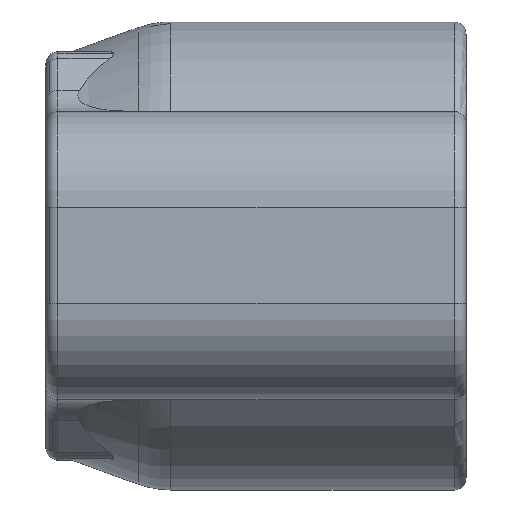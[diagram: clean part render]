
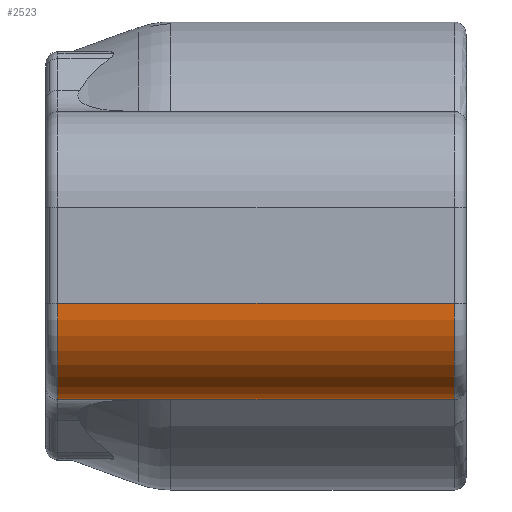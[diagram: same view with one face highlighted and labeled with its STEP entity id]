
A CAD part, top view. The second image highlights one B-rep face of the part: STEP entity #2523.
In plain terms, the highlighted cylindrical face has radius 8 mm (diameter 16 mm), a partial arc.
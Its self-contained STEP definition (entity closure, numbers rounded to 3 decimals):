
#264 = DIRECTION ( 'NONE',  ( 0., 0., 1. ) ) ;
#381 = VERTEX_POINT ( 'NONE', #6163 ) ;
#621 = EDGE_CURVE ( 'NONE', #2818, #786, #5773, .T. ) ;
#786 = VERTEX_POINT ( 'NONE', #4463 ) ;
#959 = FACE_OUTER_BOUND ( 'NONE', #5368, .T. ) ;
#1476 = AXIS2_PLACEMENT_3D ( 'NONE', #1784, #1839, #2491 ) ;
#1775 = AXIS2_PLACEMENT_3D ( 'NONE', #8683, #5584, #264 ) ;
#1784 = CARTESIAN_POINT ( 'NONE',  ( 164.981, -4., -79. ) ) ;
#1839 = DIRECTION ( 'NONE',  ( -1., 0., 0. ) ) ;
#2408 = DIRECTION ( 'NONE',  ( 1., 0., 0. ) ) ;
#2491 = DIRECTION ( 'NONE',  ( 0., 0., -1. ) ) ;
#2497 = VERTEX_POINT ( 'NONE', #4099 ) ;
#2523 = ADVANCED_FACE ( 'NONE', ( #959 ), #3412, .T. ) ;
#2673 = EDGE_CURVE ( 'NONE', #381, #2497, #6860, .T. ) ;
#2765 = CARTESIAN_POINT ( 'NONE',  ( 131.981, -4., -79. ) ) ;
#2818 = VERTEX_POINT ( 'NONE', #5273 ) ;
#2853 = VECTOR ( 'NONE', #9043, 1000. ) ;
#3150 = EDGE_CURVE ( 'NONE', #381, #2818, #9167, .T. ) ;
#3412 = CYLINDRICAL_SURFACE ( 'NONE', #1775, 8. ) ;
#4099 = CARTESIAN_POINT ( 'NONE',  ( 131.981, -4., -71. ) ) ;
#4325 = AXIS2_PLACEMENT_3D ( 'NONE', #2765, #8084, #9570 ) ;
#4463 = CARTESIAN_POINT ( 'NONE',  ( 164.981, -4., -71. ) ) ;
#4755 = EDGE_CURVE ( 'NONE', #2497, #786, #9785, .T. ) ;
#4781 = ORIENTED_EDGE ( 'NONE', *, *, #2673, .F. ) ;
#5273 = CARTESIAN_POINT ( 'NONE',  ( 164.981, -12., -79. ) ) ;
#5368 = EDGE_LOOP ( 'NONE', ( #6329, #8853, #6639, #4781 ) ) ;
#5584 = DIRECTION ( 'NONE',  ( 1., 0., 0. ) ) ;
#5773 = CIRCLE ( 'NONE', #1476, 8. ) ;
#6163 = CARTESIAN_POINT ( 'NONE',  ( 131.981, -12., -79. ) ) ;
#6329 = ORIENTED_EDGE ( 'NONE', *, *, #3150, .T. ) ;
#6410 = VECTOR ( 'NONE', #2408, 1000. ) ;
#6639 = ORIENTED_EDGE ( 'NONE', *, *, #4755, .F. ) ;
#6851 = CARTESIAN_POINT ( 'NONE',  ( 130.981, -4., -71. ) ) ;
#6860 = CIRCLE ( 'NONE', #4325, 8. ) ;
#8084 = DIRECTION ( 'NONE',  ( -1., 0., 0. ) ) ;
#8683 = CARTESIAN_POINT ( 'NONE',  ( 130.981, -4., -79. ) ) ;
#8853 = ORIENTED_EDGE ( 'NONE', *, *, #621, .T. ) ;
#9043 = DIRECTION ( 'NONE',  ( 1., 0., 0. ) ) ;
#9167 = LINE ( 'NONE', #9765, #6410 ) ;
#9570 = DIRECTION ( 'NONE',  ( 0., -0.707, 0.707 ) ) ;
#9765 = CARTESIAN_POINT ( 'NONE',  ( 130.981, -12., -79. ) ) ;
#9785 = LINE ( 'NONE', #6851, #2853 ) ;
